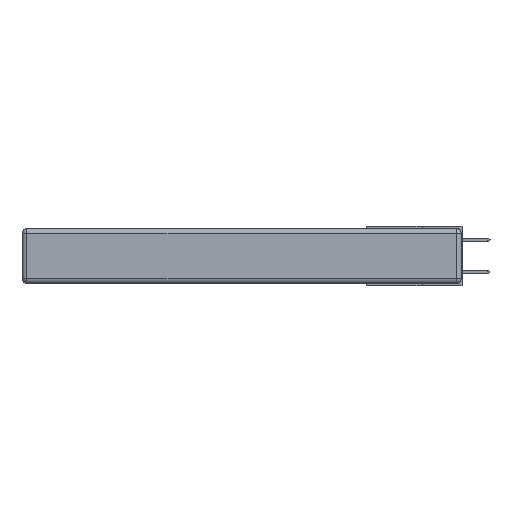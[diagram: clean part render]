
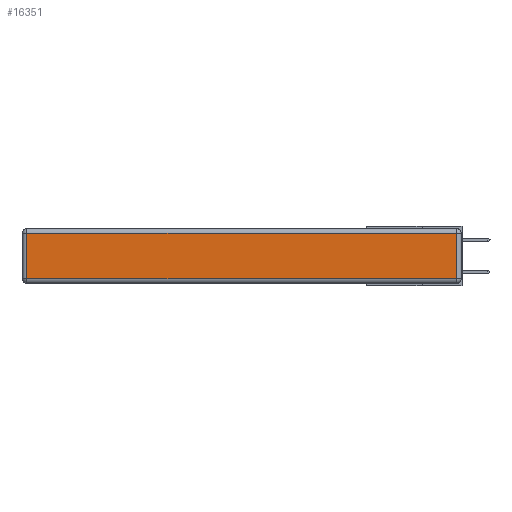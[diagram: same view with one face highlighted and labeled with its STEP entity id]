
A CAD part, left-side view. The second image highlights one B-rep face of the part: STEP entity #16351.
In plain terms, the highlighted planar face has unit normal (-1, 0, 0).
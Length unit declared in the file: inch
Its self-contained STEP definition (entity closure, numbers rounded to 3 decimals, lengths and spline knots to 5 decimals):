
#863 = DIRECTION ( 'NONE',  ( 0., 1., 0. ) ) ;
#1586 = DIRECTION ( 'NONE',  ( 0., 0., 1. ) ) ;
#3403 = FACE_OUTER_BOUND ( 'NONE', #19904, .T. ) ;
#4666 = CARTESIAN_POINT ( 'NONE',  ( 0., 0.03, -0.03 ) ) ;
#4923 = VERTEX_POINT ( 'NONE', #24748 ) ;
#5229 = ORIENTED_EDGE ( 'NONE', *, *, #19905, .T. ) ;
#5713 = CARTESIAN_POINT ( 'NONE',  ( 0., 2.72, -0.343 ) ) ;
#5831 = EDGE_CURVE ( 'NONE', #7604, #31233, #26893, .T. ) ;
#6157 = EDGE_CURVE ( 'NONE', #31233, #11114, #28797, .T. ) ;
#6354 = VECTOR ( 'NONE', #863, 39.37008 ) ;
#6681 = VECTOR ( 'NONE', #22616, 39.37008 ) ;
#7604 = VERTEX_POINT ( 'NONE', #24039 ) ;
#8204 = LINE ( 'NONE', #5713, #6681 ) ;
#8210 = CARTESIAN_POINT ( 'NONE',  ( 0., 0., -0.313 ) ) ;
#8426 = DIRECTION ( 'NONE',  ( 0., -1., 0. ) ) ;
#11114 = VERTEX_POINT ( 'NONE', #18353 ) ;
#11810 = ORIENTED_EDGE ( 'NONE', *, *, #18907, .T. ) ;
#12433 = LINE ( 'NONE', #8210, #20044 ) ;
#12486 = ORIENTED_EDGE ( 'NONE', *, *, #5831, .T. ) ;
#16351 = ADVANCED_FACE ( 'NONE', ( #3403 ), #28070, .T. ) ;
#17552 = AXIS2_PLACEMENT_3D ( 'NONE', #22919, #25484, #1586 ) ;
#18167 = CARTESIAN_POINT ( 'NONE',  ( 0., 2.75, -0.03 ) ) ;
#18353 = CARTESIAN_POINT ( 'NONE',  ( 0., 2.72, -0.03 ) ) ;
#18885 = VECTOR ( 'NONE', #24589, 39.37008 ) ;
#18907 = EDGE_CURVE ( 'NONE', #11114, #4923, #8204, .T. ) ;
#19904 = EDGE_LOOP ( 'NONE', ( #5229, #12486, #29212, #11810 ) ) ;
#19905 = EDGE_CURVE ( 'NONE', #4923, #7604, #12433, .T. ) ;
#20044 = VECTOR ( 'NONE', #8426, 39.37008 ) ;
#22616 = DIRECTION ( 'NONE',  ( 0., 0., -1. ) ) ;
#22919 = CARTESIAN_POINT ( 'NONE',  ( 0., 0., -0.343 ) ) ;
#24039 = CARTESIAN_POINT ( 'NONE',  ( 0., 0.03, -0.313 ) ) ;
#24589 = DIRECTION ( 'NONE',  ( 0., 0., 1. ) ) ;
#24748 = CARTESIAN_POINT ( 'NONE',  ( 0., 2.72, -0.313 ) ) ;
#25484 = DIRECTION ( 'NONE',  ( -1., 0., 0. ) ) ;
#26893 = LINE ( 'NONE', #27147, #18885 ) ;
#27147 = CARTESIAN_POINT ( 'NONE',  ( 0., 0.03, -0.343 ) ) ;
#28070 = PLANE ( 'NONE',  #17552 ) ;
#28797 = LINE ( 'NONE', #18167, #6354 ) ;
#29212 = ORIENTED_EDGE ( 'NONE', *, *, #6157, .T. ) ;
#31233 = VERTEX_POINT ( 'NONE', #4666 ) ;
